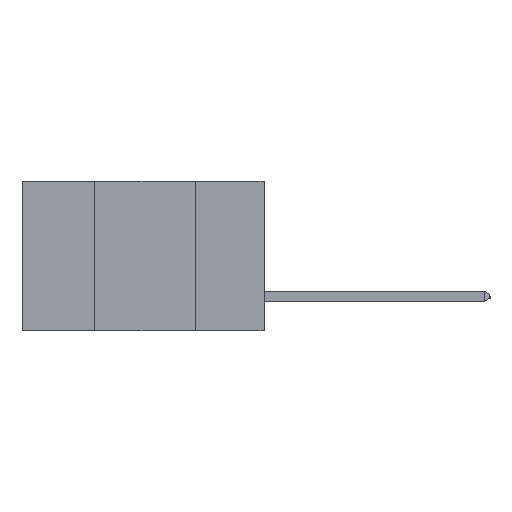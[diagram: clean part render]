
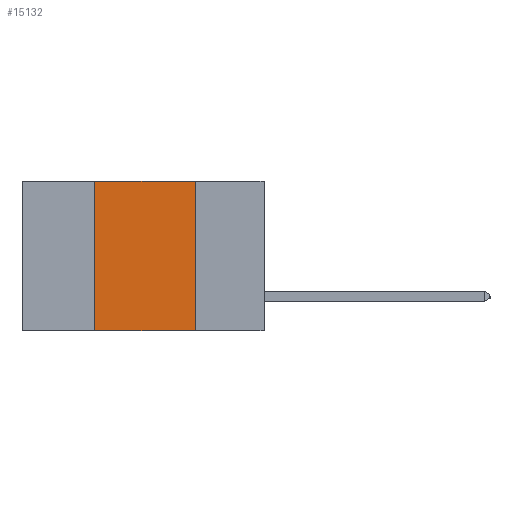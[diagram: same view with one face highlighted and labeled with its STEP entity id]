
A CAD part, left-side view. The second image highlights one B-rep face of the part: STEP entity #15132.
In plain terms, the highlighted planar face has unit normal (-1, 0, 0).
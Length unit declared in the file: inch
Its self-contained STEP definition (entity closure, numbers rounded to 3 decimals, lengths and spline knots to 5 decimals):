
#655 = LINE ( 'NONE', #20780, #11329 ) ;
#859 = DIRECTION ( 'NONE',  ( 0., 0., -1. ) ) ;
#2467 = EDGE_CURVE ( 'NONE', #6531, #18621, #26964, .T. ) ;
#2656 = FACE_OUTER_BOUND ( 'NONE', #21418, .T. ) ;
#3214 = ORIENTED_EDGE ( 'NONE', *, *, #23379, .F. ) ;
#4840 = CARTESIAN_POINT ( 'NONE',  ( 0., 0.17, 0. ) ) ;
#5101 = LINE ( 'NONE', #5151, #5783 ) ;
#5151 = CARTESIAN_POINT ( 'NONE',  ( 0., 0.6, 0. ) ) ;
#5576 = EDGE_CURVE ( 'NONE', #27013, #24849, #5101, .T. ) ;
#5783 = VECTOR ( 'NONE', #17569, 39.37008 ) ;
#6531 = VERTEX_POINT ( 'NONE', #10166 ) ;
#6617 = LINE ( 'NONE', #13855, #22453 ) ;
#7979 = CARTESIAN_POINT ( 'NONE',  ( 0., 0.42, 0. ) ) ;
#10166 = CARTESIAN_POINT ( 'NONE',  ( 0., 0.42, -0.37 ) ) ;
#10453 = DIRECTION ( 'NONE',  ( 0., -1., 0. ) ) ;
#11239 = VECTOR ( 'NONE', #10453, 39.37008 ) ;
#11329 = VECTOR ( 'NONE', #22860, 39.37008 ) ;
#13540 = DIRECTION ( 'NONE',  ( 1., 0., 0. ) ) ;
#13855 = CARTESIAN_POINT ( 'NONE',  ( 0., 0.17, 0. ) ) ;
#14828 = CARTESIAN_POINT ( 'NONE',  ( 0., 0.17, -0.37 ) ) ;
#15132 = ADVANCED_FACE ( 'NONE', ( #2656 ), #21713, .F. ) ;
#15913 = DIRECTION ( 'NONE',  ( 0., 0., -1. ) ) ;
#17569 = DIRECTION ( 'NONE',  ( 0., -1., 0. ) ) ;
#18494 = ORIENTED_EDGE ( 'NONE', *, *, #25610, .F. ) ;
#18621 = VERTEX_POINT ( 'NONE', #14828 ) ;
#19095 = CARTESIAN_POINT ( 'NONE',  ( 0., 0.6, -0.37 ) ) ;
#20456 = ORIENTED_EDGE ( 'NONE', *, *, #2467, .T. ) ;
#20780 = CARTESIAN_POINT ( 'NONE',  ( 0., 0.42, 0. ) ) ;
#21418 = EDGE_LOOP ( 'NONE', ( #18494, #24617, #3214, #20456 ) ) ;
#21713 = PLANE ( 'NONE',  #26865 ) ;
#22453 = VECTOR ( 'NONE', #15913, 39.37008 ) ;
#22860 = DIRECTION ( 'NONE',  ( 0., 0., 1. ) ) ;
#23379 = EDGE_CURVE ( 'NONE', #6531, #27013, #655, .T. ) ;
#24617 = ORIENTED_EDGE ( 'NONE', *, *, #5576, .F. ) ;
#24849 = VERTEX_POINT ( 'NONE', #4840 ) ;
#25610 = EDGE_CURVE ( 'NONE', #24849, #18621, #6617, .T. ) ;
#25837 = CARTESIAN_POINT ( 'NONE',  ( 0., 0.6, 0. ) ) ;
#26865 = AXIS2_PLACEMENT_3D ( 'NONE', #25837, #13540, #859 ) ;
#26964 = LINE ( 'NONE', #19095, #11239 ) ;
#27013 = VERTEX_POINT ( 'NONE', #7979 ) ;
